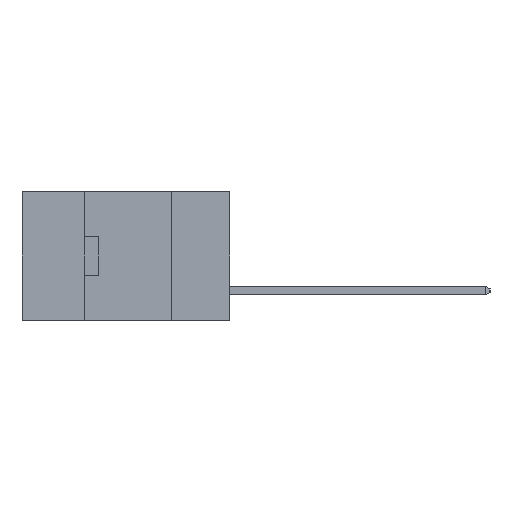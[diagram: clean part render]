
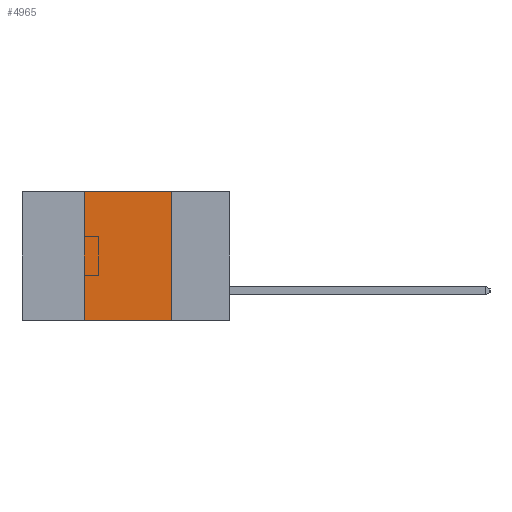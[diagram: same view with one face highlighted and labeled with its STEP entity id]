
A CAD part, left-side view. The second image highlights one B-rep face of the part: STEP entity #4965.
In plain terms, the highlighted planar face has unit normal (-1, 0, 0).
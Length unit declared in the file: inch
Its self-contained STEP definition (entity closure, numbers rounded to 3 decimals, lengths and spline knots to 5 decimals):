
#42 = CARTESIAN_POINT ( 'NONE',  ( 0., 0.42, 0. ) ) ;
#90 = VECTOR ( 'NONE', #8117, 39.37008 ) ;
#113 = LINE ( 'NONE', #26372, #11397 ) ;
#657 = CARTESIAN_POINT ( 'NONE',  ( 0., 0.17, 0. ) ) ;
#770 = DIRECTION ( 'NONE',  ( 0., 0., -1. ) ) ;
#1382 = DIRECTION ( 'NONE',  ( 0., 0., 1. ) ) ;
#2449 = CARTESIAN_POINT ( 'NONE',  ( 0., 0.17, -0.37 ) ) ;
#3104 = ORIENTED_EDGE ( 'NONE', *, *, #20568, .F. ) ;
#3451 = ORIENTED_EDGE ( 'NONE', *, *, #11924, .F. ) ;
#4354 = ORIENTED_EDGE ( 'NONE', *, *, #17519, .T. ) ;
#4965 = ADVANCED_FACE ( 'NONE', ( #5149 ), #14511, .F. ) ;
#5149 = FACE_OUTER_BOUND ( 'NONE', #26105, .T. ) ;
#5747 = LINE ( 'NONE', #5969, #90 ) ;
#5969 = CARTESIAN_POINT ( 'NONE',  ( 0., 0.6, 0. ) ) ;
#6502 = LINE ( 'NONE', #21209, #21907 ) ;
#7625 = VERTEX_POINT ( 'NONE', #657 ) ;
#8117 = DIRECTION ( 'NONE',  ( 0., -1., 0. ) ) ;
#9711 = ORIENTED_EDGE ( 'NONE', *, *, #19463, .F. ) ;
#11397 = VECTOR ( 'NONE', #1382, 39.37008 ) ;
#11924 = EDGE_CURVE ( 'NONE', #15548, #7625, #5747, .T. ) ;
#14028 = VERTEX_POINT ( 'NONE', #25327 ) ;
#14394 = DIRECTION ( 'NONE',  ( 0., 0., -1. ) ) ;
#14420 = DIRECTION ( 'NONE',  ( 1., 0., 0. ) ) ;
#14511 = PLANE ( 'NONE',  #22459 ) ;
#14605 = CARTESIAN_POINT ( 'NONE',  ( 0., 0.6, 0. ) ) ;
#14743 = VERTEX_POINT ( 'NONE', #2449 ) ;
#15548 = VERTEX_POINT ( 'NONE', #42 ) ;
#17519 = EDGE_CURVE ( 'NONE', #14028, #14743, #6502, .T. ) ;
#17549 = CARTESIAN_POINT ( 'NONE',  ( 0., 0.17, -0.37 ) ) ;
#19463 = EDGE_CURVE ( 'NONE', #14028, #15548, #113, .T. ) ;
#20166 = VECTOR ( 'NONE', #770, 39.37008 ) ;
#20568 = EDGE_CURVE ( 'NONE', #7625, #14743, #25565, .T. ) ;
#21209 = CARTESIAN_POINT ( 'NONE',  ( 0., 0.6, -0.37 ) ) ;
#21907 = VECTOR ( 'NONE', #23286, 39.37008 ) ;
#22459 = AXIS2_PLACEMENT_3D ( 'NONE', #14605, #14420, #14394 ) ;
#23286 = DIRECTION ( 'NONE',  ( 0., -1., 0. ) ) ;
#25327 = CARTESIAN_POINT ( 'NONE',  ( 0., 0.42, -0.37 ) ) ;
#25565 = LINE ( 'NONE', #17549, #20166 ) ;
#26105 = EDGE_LOOP ( 'NONE', ( #3104, #3451, #9711, #4354 ) ) ;
#26372 = CARTESIAN_POINT ( 'NONE',  ( 0., 0.42, -0.37 ) ) ;
